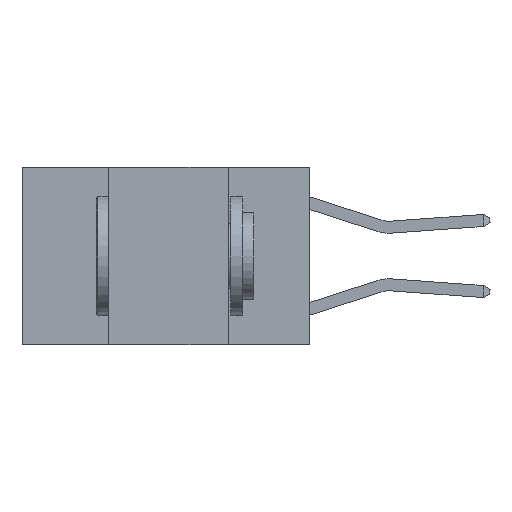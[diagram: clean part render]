
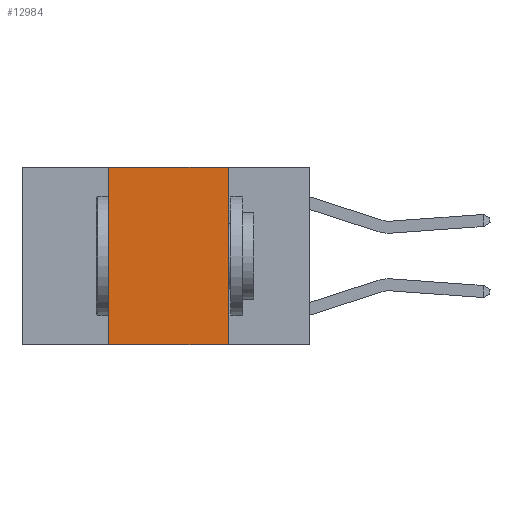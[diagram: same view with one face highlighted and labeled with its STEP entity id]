
A CAD part, left-side view. The second image highlights one B-rep face of the part: STEP entity #12984.
In plain terms, the highlighted planar face has unit normal (-1, 0, 0).
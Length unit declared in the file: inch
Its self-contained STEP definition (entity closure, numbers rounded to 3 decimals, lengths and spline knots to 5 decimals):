
#1847 = CARTESIAN_POINT ( 'NONE',  ( 0., 0.6, 0. ) ) ;
#1975 = DIRECTION ( 'NONE',  ( 0., -1., 0. ) ) ;
#2470 = EDGE_CURVE ( 'NONE', #19467, #22440, #10491, .T. ) ;
#2609 = CARTESIAN_POINT ( 'NONE',  ( 0., 0.42, -0.37 ) ) ;
#2884 = DIRECTION ( 'NONE',  ( 1., 0., 0. ) ) ;
#3265 = DIRECTION ( 'NONE',  ( 0., 0., -1. ) ) ;
#3462 = ORIENTED_EDGE ( 'NONE', *, *, #2470, .F. ) ;
#3748 = LINE ( 'NONE', #1847, #23887 ) ;
#5049 = ORIENTED_EDGE ( 'NONE', *, *, #19367, .T. ) ;
#5452 = VECTOR ( 'NONE', #8580, 39.37008 ) ;
#5564 = VECTOR ( 'NONE', #17761, 39.37008 ) ;
#5675 = CARTESIAN_POINT ( 'NONE',  ( 0., 0.17, -0.37 ) ) ;
#6125 = DIRECTION ( 'NONE',  ( 0., -1., 0. ) ) ;
#6160 = VECTOR ( 'NONE', #6125, 39.37008 ) ;
#8090 = LINE ( 'NONE', #19919, #5564 ) ;
#8190 = VERTEX_POINT ( 'NONE', #22015 ) ;
#8278 = LINE ( 'NONE', #11845, #6160 ) ;
#8580 = DIRECTION ( 'NONE',  ( 0., 0., -1. ) ) ;
#9207 = VERTEX_POINT ( 'NONE', #2609 ) ;
#10491 = LINE ( 'NONE', #10615, #5452 ) ;
#10615 = CARTESIAN_POINT ( 'NONE',  ( 0., 0.17, 0. ) ) ;
#11763 = EDGE_CURVE ( 'NONE', #9207, #8190, #8090, .T. ) ;
#11845 = CARTESIAN_POINT ( 'NONE',  ( 0., 0.6, -0.37 ) ) ;
#12554 = CARTESIAN_POINT ( 'NONE',  ( 0., 0.6, 0. ) ) ;
#12856 = CARTESIAN_POINT ( 'NONE',  ( 0., 0.17, 0. ) ) ;
#12984 = ADVANCED_FACE ( 'NONE', ( #14580 ), #16637, .F. ) ;
#13170 = EDGE_CURVE ( 'NONE', #8190, #19467, #3748, .T. ) ;
#14580 = FACE_OUTER_BOUND ( 'NONE', #21671, .T. ) ;
#15348 = AXIS2_PLACEMENT_3D ( 'NONE', #12554, #2884, #3265 ) ;
#16637 = PLANE ( 'NONE',  #15348 ) ;
#16903 = ORIENTED_EDGE ( 'NONE', *, *, #11763, .F. ) ;
#17192 = ORIENTED_EDGE ( 'NONE', *, *, #13170, .F. ) ;
#17761 = DIRECTION ( 'NONE',  ( 0., 0., 1. ) ) ;
#19367 = EDGE_CURVE ( 'NONE', #9207, #22440, #8278, .T. ) ;
#19467 = VERTEX_POINT ( 'NONE', #12856 ) ;
#19919 = CARTESIAN_POINT ( 'NONE',  ( 0., 0.42, 0. ) ) ;
#21671 = EDGE_LOOP ( 'NONE', ( #3462, #17192, #16903, #5049 ) ) ;
#22015 = CARTESIAN_POINT ( 'NONE',  ( 0., 0.42, 0. ) ) ;
#22440 = VERTEX_POINT ( 'NONE', #5675 ) ;
#23887 = VECTOR ( 'NONE', #1975, 39.37008 ) ;
